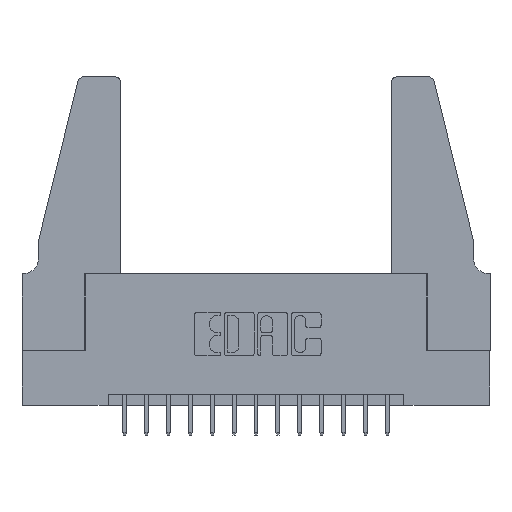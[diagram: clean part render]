
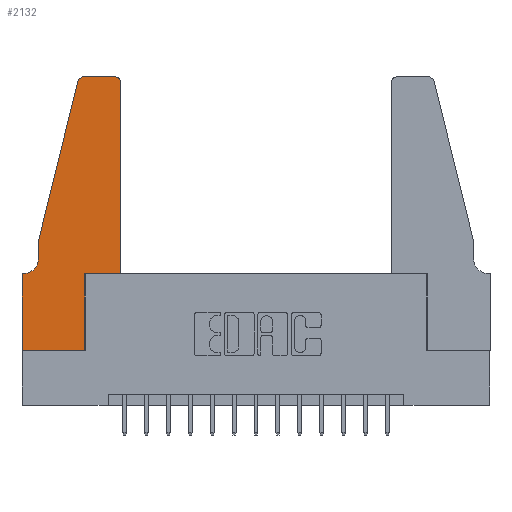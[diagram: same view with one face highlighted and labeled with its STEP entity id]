
A CAD part, top view. The second image highlights one B-rep face of the part: STEP entity #2132.
In plain terms, the highlighted planar face has unit normal (0, 0, 1).
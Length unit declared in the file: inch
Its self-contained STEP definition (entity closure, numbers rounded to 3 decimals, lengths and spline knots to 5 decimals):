
#92 = DIRECTION ( 'NONE',  ( 1., 0., 0. ) ) ;
#260 = CARTESIAN_POINT ( 'NONE',  ( 0.0055, 0.42, 0.37 ) ) ;
#403 = DIRECTION ( 'NONE',  ( 1., 0., 0. ) ) ;
#479 = CIRCLE ( 'NONE', #13162, 0.03 ) ;
#538 = VECTOR ( 'NONE', #7936, 39.37008 ) ;
#614 = VERTEX_POINT ( 'NONE', #12609 ) ;
#687 = EDGE_CURVE ( 'NONE', #6645, #11002, #6221, .T. ) ;
#781 = EDGE_CURVE ( 'NONE', #12778, #12105, #11288, .T. ) ;
#902 = AXIS2_PLACEMENT_3D ( 'NONE', #6875, #10547, #403 ) ;
#1047 = CARTESIAN_POINT ( 'NONE',  ( 0.4205, 1.25, 0.37 ) ) ;
#1383 = ORIENTED_EDGE ( 'NONE', *, *, #8790, .T. ) ;
#1392 = CARTESIAN_POINT ( 'NONE',  ( 0.0755, 0.5, 0.37 ) ) ;
#1508 = DIRECTION ( 'NONE',  ( 1., 0., 0. ) ) ;
#1834 = EDGE_LOOP ( 'NONE', ( #8157, #3382, #13418, #5283, #9457, #1383, #11745, #15366, #14057, #9784, #12329, #7292 ) ) ;
#2101 = DIRECTION ( 'NONE',  ( 0., -1., 0. ) ) ;
#2132 = ADVANCED_FACE ( 'NONE', ( #9114 ), #7895, .T. ) ;
#2184 = LINE ( 'NONE', #13262, #5746 ) ;
#2751 = DIRECTION ( 'NONE',  ( -0.239, -0.971, 0. ) ) ;
#2779 = DIRECTION ( 'NONE',  ( 0., 0., 1. ) ) ;
#3382 = ORIENTED_EDGE ( 'NONE', *, *, #687, .T. ) ;
#3588 = DIRECTION ( 'NONE',  ( 0., 1., 0. ) ) ;
#3854 = DIRECTION ( 'NONE',  ( 0., 0., 1. ) ) ;
#3856 = CARTESIAN_POINT ( 'NONE',  ( 0.2605, 1.25, 0.37 ) ) ;
#3990 = DIRECTION ( 'NONE',  ( 1., 0., 0. ) ) ;
#4039 = VERTEX_POINT ( 'NONE', #9339 ) ;
#4470 = CARTESIAN_POINT ( 'NONE',  ( 0., 0.35, 0.37 ) ) ;
#4751 = CARTESIAN_POINT ( 'NONE',  ( 0.2865, 0.35, 0.37 ) ) ;
#4789 = CARTESIAN_POINT ( 'NONE',  ( 0.284, 1.25, 0.37 ) ) ;
#4923 = EDGE_CURVE ( 'NONE', #4039, #12778, #10742, .T. ) ;
#5150 = VERTEX_POINT ( 'NONE', #15292 ) ;
#5183 = CARTESIAN_POINT ( 'NONE',  ( 0.4205, 1.22, 0.37 ) ) ;
#5283 = ORIENTED_EDGE ( 'NONE', *, *, #15174, .T. ) ;
#5578 = VECTOR ( 'NONE', #13783, 39.37008 ) ;
#5593 = DIRECTION ( 'NONE',  ( -1., 0., 0. ) ) ;
#5746 = VECTOR ( 'NONE', #14662, 39.37008 ) ;
#6102 = VECTOR ( 'NONE', #15007, 39.37008 ) ;
#6169 = VERTEX_POINT ( 'NONE', #1047 ) ;
#6221 = CIRCLE ( 'NONE', #902, 0.03 ) ;
#6264 = CARTESIAN_POINT ( 'NONE',  ( 0.4505, 0.35, 0.37 ) ) ;
#6645 = VERTEX_POINT ( 'NONE', #4789 ) ;
#6826 = CARTESIAN_POINT ( 'NONE',  ( 0.0755, 0.5, 0.37 ) ) ;
#6871 = VECTOR ( 'NONE', #10168, 39.37008 ) ;
#6875 = CARTESIAN_POINT ( 'NONE',  ( 0.284, 1.22, 0.37 ) ) ;
#7048 = EDGE_CURVE ( 'NONE', #13893, #7801, #15553, .T. ) ;
#7292 = ORIENTED_EDGE ( 'NONE', *, *, #13586, .T. ) ;
#7486 = CARTESIAN_POINT ( 'NONE',  ( 0., 0., 0.37 ) ) ;
#7801 = VERTEX_POINT ( 'NONE', #10977 ) ;
#7895 = PLANE ( 'NONE',  #10488 ) ;
#7936 = DIRECTION ( 'NONE',  ( -1., 0., 0. ) ) ;
#8157 = ORIENTED_EDGE ( 'NONE', *, *, #15300, .T. ) ;
#8285 = EDGE_CURVE ( 'NONE', #11002, #11964, #13986, .T. ) ;
#8785 = LINE ( 'NONE', #12548, #5578 ) ;
#8790 = EDGE_CURVE ( 'NONE', #7801, #14738, #9225, .T. ) ;
#8844 = VECTOR ( 'NONE', #2101, 39.37008 ) ;
#9114 = FACE_OUTER_BOUND ( 'NONE', #1834, .T. ) ;
#9225 = LINE ( 'NONE', #14208, #538 ) ;
#9339 = CARTESIAN_POINT ( 'NONE',  ( 0.2865, 0., 0.37 ) ) ;
#9457 = ORIENTED_EDGE ( 'NONE', *, *, #7048, .T. ) ;
#9784 = ORIENTED_EDGE ( 'NONE', *, *, #781, .T. ) ;
#9891 = EDGE_CURVE ( 'NONE', #14738, #5150, #13788, .T. ) ;
#10168 = DIRECTION ( 'NONE',  ( -1., 0., 0. ) ) ;
#10488 = AXIS2_PLACEMENT_3D ( 'NONE', #14086, #2779, #1508 ) ;
#10547 = DIRECTION ( 'NONE',  ( 0., 0., 1. ) ) ;
#10742 = LINE ( 'NONE', #4751, #14977 ) ;
#10977 = CARTESIAN_POINT ( 'NONE',  ( 0.0055, 0.35, 0.37 ) ) ;
#11002 = VERTEX_POINT ( 'NONE', #14289 ) ;
#11257 = CARTESIAN_POINT ( 'NONE',  ( 0.2865, 0.35, 0.37 ) ) ;
#11288 = LINE ( 'NONE', #11515, #11757 ) ;
#11313 = EDGE_CURVE ( 'NONE', #5150, #4039, #2184, .T. ) ;
#11366 = AXIS2_PLACEMENT_3D ( 'NONE', #260, #11885, #5593 ) ;
#11515 = CARTESIAN_POINT ( 'NONE',  ( 0.4505, 0.35, 0.37 ) ) ;
#11745 = ORIENTED_EDGE ( 'NONE', *, *, #9891, .T. ) ;
#11757 = VECTOR ( 'NONE', #3990, 39.37008 ) ;
#11885 = DIRECTION ( 'NONE',  ( 0., 0., -1. ) ) ;
#11964 = VERTEX_POINT ( 'NONE', #6826 ) ;
#12105 = VERTEX_POINT ( 'NONE', #12551 ) ;
#12329 = ORIENTED_EDGE ( 'NONE', *, *, #15158, .T. ) ;
#12548 = CARTESIAN_POINT ( 'NONE',  ( 0.0755, 0.5, 0.37 ) ) ;
#12551 = CARTESIAN_POINT ( 'NONE',  ( 0.4505, 0.35, 0.37 ) ) ;
#12609 = CARTESIAN_POINT ( 'NONE',  ( 0.4505, 1.22, 0.37 ) ) ;
#12712 = LINE ( 'NONE', #3856, #6871 ) ;
#12778 = VERTEX_POINT ( 'NONE', #11257 ) ;
#13162 = AXIS2_PLACEMENT_3D ( 'NONE', #5183, #3854, #92 ) ;
#13262 = CARTESIAN_POINT ( 'NONE',  ( 0., 0., 0.37 ) ) ;
#13418 = ORIENTED_EDGE ( 'NONE', *, *, #8285, .T. ) ;
#13586 = EDGE_CURVE ( 'NONE', #614, #6169, #479, .T. ) ;
#13743 = VECTOR ( 'NONE', #2751, 39.37008 ) ;
#13783 = DIRECTION ( 'NONE',  ( 0., -1., 0. ) ) ;
#13788 = LINE ( 'NONE', #7486, #8844 ) ;
#13893 = VERTEX_POINT ( 'NONE', #15552 ) ;
#13986 = LINE ( 'NONE', #1392, #13743 ) ;
#14057 = ORIENTED_EDGE ( 'NONE', *, *, #4923, .T. ) ;
#14086 = CARTESIAN_POINT ( 'NONE',  ( 0., 0.35, 0.37 ) ) ;
#14208 = CARTESIAN_POINT ( 'NONE',  ( 0.0755, 0.35, 0.37 ) ) ;
#14289 = CARTESIAN_POINT ( 'NONE',  ( 0.25487, 1.22718, 0.37 ) ) ;
#14662 = DIRECTION ( 'NONE',  ( 1., 0., 0. ) ) ;
#14738 = VERTEX_POINT ( 'NONE', #4470 ) ;
#14977 = VECTOR ( 'NONE', #3588, 39.37008 ) ;
#15007 = DIRECTION ( 'NONE',  ( 0., 1., 0. ) ) ;
#15158 = EDGE_CURVE ( 'NONE', #12105, #614, #16245, .T. ) ;
#15174 = EDGE_CURVE ( 'NONE', #11964, #13893, #8785, .T. ) ;
#15292 = CARTESIAN_POINT ( 'NONE',  ( 0., 0., 0.37 ) ) ;
#15300 = EDGE_CURVE ( 'NONE', #6169, #6645, #12712, .T. ) ;
#15366 = ORIENTED_EDGE ( 'NONE', *, *, #11313, .T. ) ;
#15552 = CARTESIAN_POINT ( 'NONE',  ( 0.0755, 0.42, 0.37 ) ) ;
#15553 = CIRCLE ( 'NONE', #11366, 0.07 ) ;
#16245 = LINE ( 'NONE', #6264, #6102 ) ;
